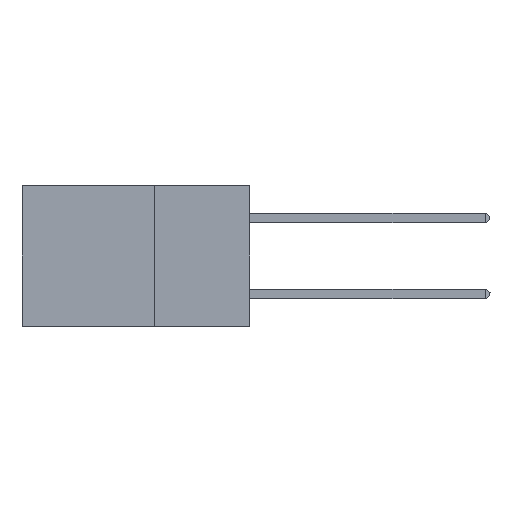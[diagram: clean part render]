
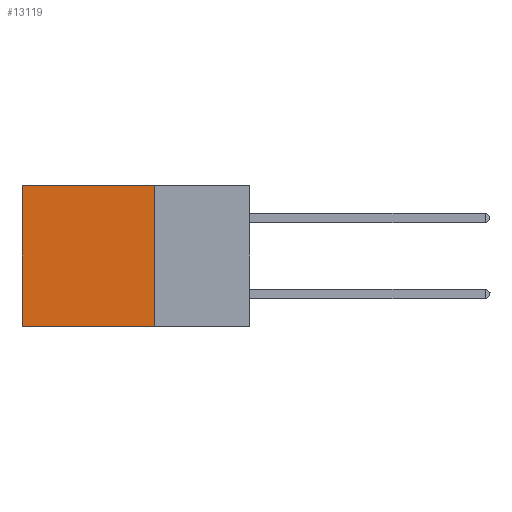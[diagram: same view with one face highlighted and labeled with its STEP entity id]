
A CAD part, left-side view. The second image highlights one B-rep face of the part: STEP entity #13119.
In plain terms, the highlighted planar face has unit normal (-1, 0, 0).
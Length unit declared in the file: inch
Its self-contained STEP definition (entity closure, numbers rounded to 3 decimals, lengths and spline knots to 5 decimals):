
#956 = VECTOR ( 'NONE', #14972, 39.37008 ) ;
#1183 = EDGE_CURVE ( 'NONE', #14494, #11672, #21548, .T. ) ;
#1505 = LINE ( 'NONE', #12733, #19245 ) ;
#1746 = CARTESIAN_POINT ( 'NONE',  ( 0.2875, 0.25, 0. ) ) ;
#3312 = ORIENTED_EDGE ( 'NONE', *, *, #18522, .T. ) ;
#4704 = VECTOR ( 'NONE', #19459, 39.37008 ) ;
#5303 = CARTESIAN_POINT ( 'NONE',  ( 0.2875, 0.6, -0.37 ) ) ;
#5681 = AXIS2_PLACEMENT_3D ( 'NONE', #28356, #6294, #23351 ) ;
#6294 = DIRECTION ( 'NONE',  ( 1., 0., 0. ) ) ;
#7751 = ORIENTED_EDGE ( 'NONE', *, *, #13696, .F. ) ;
#8192 = LINE ( 'NONE', #1746, #27074 ) ;
#10659 = DIRECTION ( 'NONE',  ( 0., 0., -1. ) ) ;
#10663 = PLANE ( 'NONE',  #5681 ) ;
#11144 = CARTESIAN_POINT ( 'NONE',  ( 0.2875, 0.6, 0. ) ) ;
#11672 = VERTEX_POINT ( 'NONE', #5303 ) ;
#12733 = CARTESIAN_POINT ( 'NONE',  ( 0.2875, 0.6, 0. ) ) ;
#13119 = ADVANCED_FACE ( 'NONE', ( #28216 ), #10663, .F. ) ;
#13696 = EDGE_CURVE ( 'NONE', #15458, #14494, #8192, .T. ) ;
#14494 = VERTEX_POINT ( 'NONE', #21710 ) ;
#14942 = LINE ( 'NONE', #21659, #4704 ) ;
#14972 = DIRECTION ( 'NONE',  ( 0., 1., 0. ) ) ;
#15458 = VERTEX_POINT ( 'NONE', #15595 ) ;
#15595 = CARTESIAN_POINT ( 'NONE',  ( 0.2875, 0.25, 0. ) ) ;
#16857 = ORIENTED_EDGE ( 'NONE', *, *, #1183, .F. ) ;
#17154 = CARTESIAN_POINT ( 'NONE',  ( 0.2875, 0.25, -0.37 ) ) ;
#18038 = EDGE_LOOP ( 'NONE', ( #3312, #16857, #7751, #27899 ) ) ;
#18522 = EDGE_CURVE ( 'NONE', #24398, #11672, #1505, .T. ) ;
#19245 = VECTOR ( 'NONE', #21624, 39.37008 ) ;
#19459 = DIRECTION ( 'NONE',  ( 0., 1., 0. ) ) ;
#21548 = LINE ( 'NONE', #17154, #956 ) ;
#21624 = DIRECTION ( 'NONE',  ( 0., 0., -1. ) ) ;
#21659 = CARTESIAN_POINT ( 'NONE',  ( 0.2875, 0.25, 0. ) ) ;
#21710 = CARTESIAN_POINT ( 'NONE',  ( 0.2875, 0.25, -0.37 ) ) ;
#23351 = DIRECTION ( 'NONE',  ( 0., 0., -1. ) ) ;
#24398 = VERTEX_POINT ( 'NONE', #11144 ) ;
#25662 = EDGE_CURVE ( 'NONE', #15458, #24398, #14942, .T. ) ;
#27074 = VECTOR ( 'NONE', #10659, 39.37008 ) ;
#27899 = ORIENTED_EDGE ( 'NONE', *, *, #25662, .T. ) ;
#28216 = FACE_OUTER_BOUND ( 'NONE', #18038, .T. ) ;
#28356 = CARTESIAN_POINT ( 'NONE',  ( 0.2875, 0.25, 0. ) ) ;
